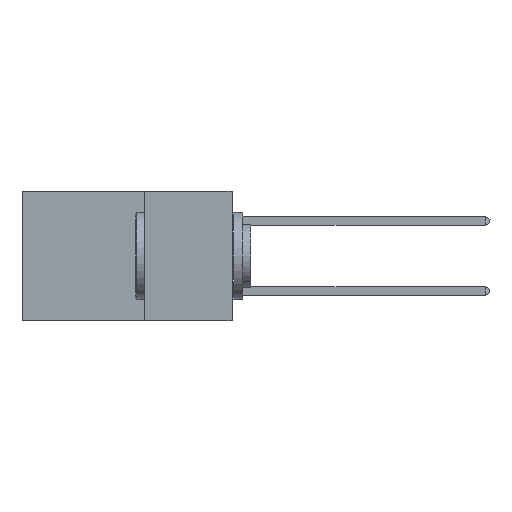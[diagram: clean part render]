
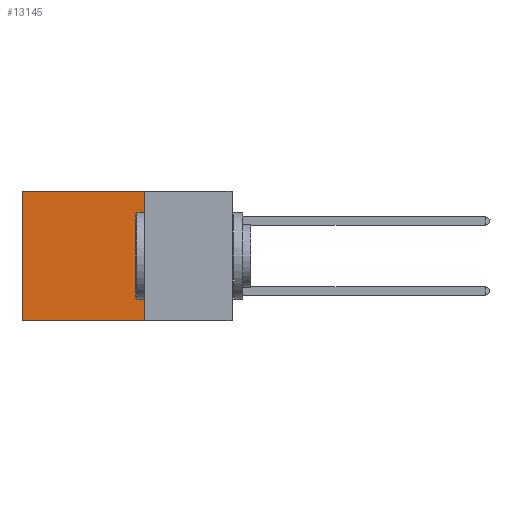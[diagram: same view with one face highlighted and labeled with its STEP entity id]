
A CAD part, left-side view. The second image highlights one B-rep face of the part: STEP entity #13145.
In plain terms, the highlighted planar face has unit normal (-1, 0, 0).
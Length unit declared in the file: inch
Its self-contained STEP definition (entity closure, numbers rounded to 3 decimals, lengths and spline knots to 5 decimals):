
#7 = DIRECTION ( 'NONE',  ( 0., 0., -1. ) ) ;
#2078 = EDGE_CURVE ( 'NONE', #24406, #18758, #17449, .T. ) ;
#2410 = ORIENTED_EDGE ( 'NONE', *, *, #2078, .F. ) ;
#2958 = CARTESIAN_POINT ( 'NONE',  ( 0.2875, 0.25, 0. ) ) ;
#6070 = DIRECTION ( 'NONE',  ( 0., 1., 0. ) ) ;
#6244 = EDGE_CURVE ( 'NONE', #19325, #14069, #15528, .T. ) ;
#7494 = CARTESIAN_POINT ( 'NONE',  ( 0.2875, 0.6, -0.37 ) ) ;
#8521 = PLANE ( 'NONE',  #25340 ) ;
#8524 = CARTESIAN_POINT ( 'NONE',  ( 0.2875, 0.25, 0. ) ) ;
#9865 = VECTOR ( 'NONE', #6070, 39.37008 ) ;
#11980 = ORIENTED_EDGE ( 'NONE', *, *, #19565, .T. ) ;
#12518 = CARTESIAN_POINT ( 'NONE',  ( 0.2875, 0.25, -0.37 ) ) ;
#13145 = ADVANCED_FACE ( 'NONE', ( #18598 ), #8521, .F. ) ;
#14069 = VERTEX_POINT ( 'NONE', #22557 ) ;
#15036 = DIRECTION ( 'NONE',  ( 1., 0., 0. ) ) ;
#15130 = CARTESIAN_POINT ( 'NONE',  ( 0.2875, 0.25, 0. ) ) ;
#15336 = VECTOR ( 'NONE', #22107, 39.37008 ) ;
#15528 = LINE ( 'NONE', #8524, #9865 ) ;
#16777 = VECTOR ( 'NONE', #24652, 39.37008 ) ;
#17449 = LINE ( 'NONE', #24737, #16777 ) ;
#17762 = CARTESIAN_POINT ( 'NONE',  ( 0.2875, 0.6, 0. ) ) ;
#17784 = ORIENTED_EDGE ( 'NONE', *, *, #6244, .T. ) ;
#18331 = LINE ( 'NONE', #2958, #15336 ) ;
#18598 = FACE_OUTER_BOUND ( 'NONE', #20128, .T. ) ;
#18758 = VERTEX_POINT ( 'NONE', #7494 ) ;
#19325 = VERTEX_POINT ( 'NONE', #24971 ) ;
#19491 = DIRECTION ( 'NONE',  ( 0., 0., -1. ) ) ;
#19565 = EDGE_CURVE ( 'NONE', #14069, #18758, #27095, .T. ) ;
#20128 = EDGE_LOOP ( 'NONE', ( #11980, #2410, #26103, #17784 ) ) ;
#21735 = EDGE_CURVE ( 'NONE', #19325, #24406, #18331, .T. ) ;
#22107 = DIRECTION ( 'NONE',  ( 0., 0., -1. ) ) ;
#22482 = VECTOR ( 'NONE', #19491, 39.37008 ) ;
#22557 = CARTESIAN_POINT ( 'NONE',  ( 0.2875, 0.6, 0. ) ) ;
#24406 = VERTEX_POINT ( 'NONE', #12518 ) ;
#24652 = DIRECTION ( 'NONE',  ( 0., 1., 0. ) ) ;
#24737 = CARTESIAN_POINT ( 'NONE',  ( 0.2875, 0.25, -0.37 ) ) ;
#24971 = CARTESIAN_POINT ( 'NONE',  ( 0.2875, 0.25, 0. ) ) ;
#25340 = AXIS2_PLACEMENT_3D ( 'NONE', #15130, #15036, #7 ) ;
#26103 = ORIENTED_EDGE ( 'NONE', *, *, #21735, .F. ) ;
#27095 = LINE ( 'NONE', #17762, #22482 ) ;
